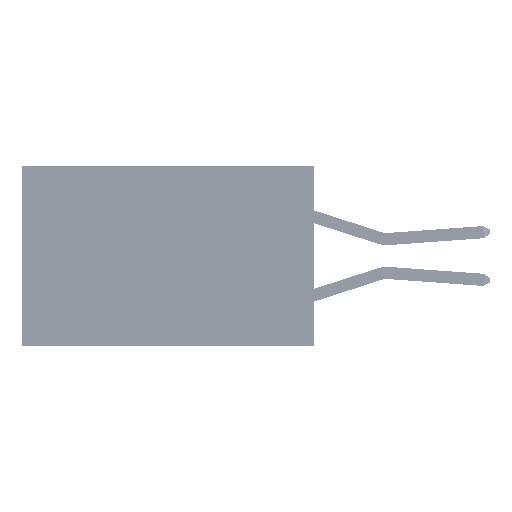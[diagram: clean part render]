
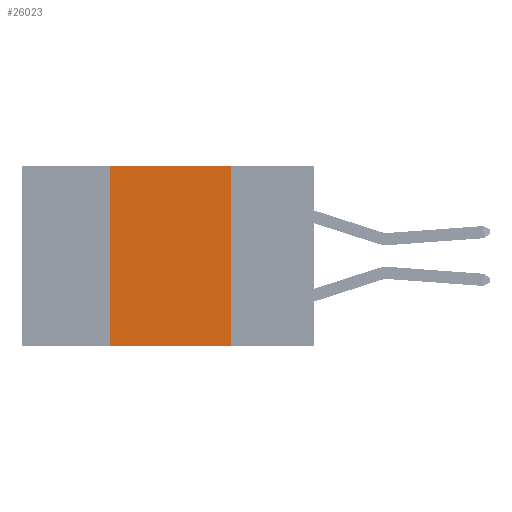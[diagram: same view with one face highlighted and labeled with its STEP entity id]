
A CAD part, left-side view. The second image highlights one B-rep face of the part: STEP entity #26023.
In plain terms, the highlighted planar face has unit normal (-1, 0, 0).
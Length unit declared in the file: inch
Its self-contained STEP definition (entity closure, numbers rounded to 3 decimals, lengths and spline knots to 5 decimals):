
#2505 = DIRECTION ( 'NONE',  ( 0., -1., 0. ) ) ;
#2664 = VERTEX_POINT ( 'NONE', #27035 ) ;
#3651 = CARTESIAN_POINT ( 'NONE',  ( 0., 0.6, 0. ) ) ;
#4185 = VECTOR ( 'NONE', #14669, 39.37008 ) ;
#7440 = DIRECTION ( 'NONE',  ( 0., 0., -1. ) ) ;
#7669 = CARTESIAN_POINT ( 'NONE',  ( 0., 0.17, -0.37 ) ) ;
#8292 = DIRECTION ( 'NONE',  ( 0., 0., -1. ) ) ;
#10336 = ORIENTED_EDGE ( 'NONE', *, *, #44571, .F. ) ;
#11085 = CARTESIAN_POINT ( 'NONE',  ( 0., 0.17, 0. ) ) ;
#11935 = VECTOR ( 'NONE', #41525, 39.37008 ) ;
#14669 = DIRECTION ( 'NONE',  ( 0., 0., 1. ) ) ;
#22605 = PLANE ( 'NONE',  #46366 ) ;
#24208 = FACE_OUTER_BOUND ( 'NONE', #46485, .T. ) ;
#24449 = LINE ( 'NONE', #25984, #4185 ) ;
#24618 = VECTOR ( 'NONE', #2505, 39.37008 ) ;
#25378 = VERTEX_POINT ( 'NONE', #7669 ) ;
#25517 = CARTESIAN_POINT ( 'NONE',  ( 0., 0.42, -0.37 ) ) ;
#25984 = CARTESIAN_POINT ( 'NONE',  ( 0., 0.42, 0. ) ) ;
#26023 = ADVANCED_FACE ( 'NONE', ( #24208 ), #22605, .F. ) ;
#27035 = CARTESIAN_POINT ( 'NONE',  ( 0., 0.42, 0. ) ) ;
#28756 = EDGE_CURVE ( 'NONE', #37394, #25378, #43657, .T. ) ;
#30022 = ORIENTED_EDGE ( 'NONE', *, *, #44798, .F. ) ;
#30258 = DIRECTION ( 'NONE',  ( 1., 0., 0. ) ) ;
#31083 = CARTESIAN_POINT ( 'NONE',  ( 0., 0.17, 0. ) ) ;
#32158 = LINE ( 'NONE', #37714, #11935 ) ;
#37394 = VERTEX_POINT ( 'NONE', #25517 ) ;
#37714 = CARTESIAN_POINT ( 'NONE',  ( 0., 0.6, 0. ) ) ;
#40103 = ORIENTED_EDGE ( 'NONE', *, *, #45306, .F. ) ;
#41525 = DIRECTION ( 'NONE',  ( 0., -1., 0. ) ) ;
#41918 = ORIENTED_EDGE ( 'NONE', *, *, #28756, .T. ) ;
#43657 = LINE ( 'NONE', #48127, #24618 ) ;
#44067 = LINE ( 'NONE', #31083, #46475 ) ;
#44571 = EDGE_CURVE ( 'NONE', #37394, #2664, #24449, .T. ) ;
#44798 = EDGE_CURVE ( 'NONE', #45318, #25378, #44067, .T. ) ;
#45306 = EDGE_CURVE ( 'NONE', #2664, #45318, #32158, .T. ) ;
#45318 = VERTEX_POINT ( 'NONE', #11085 ) ;
#46366 = AXIS2_PLACEMENT_3D ( 'NONE', #3651, #30258, #7440 ) ;
#46475 = VECTOR ( 'NONE', #8292, 39.37008 ) ;
#46485 = EDGE_LOOP ( 'NONE', ( #30022, #40103, #10336, #41918 ) ) ;
#48127 = CARTESIAN_POINT ( 'NONE',  ( 0., 0.6, -0.37 ) ) ;
